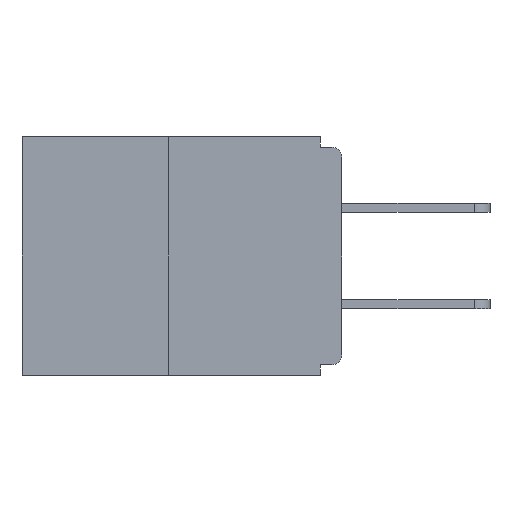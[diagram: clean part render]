
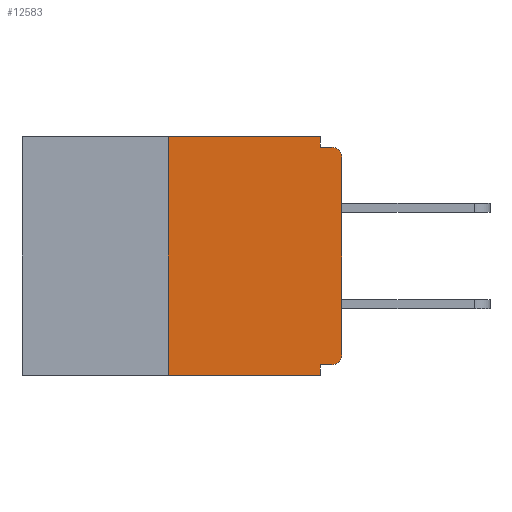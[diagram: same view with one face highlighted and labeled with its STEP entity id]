
A CAD part, left-side view. The second image highlights one B-rep face of the part: STEP entity #12583.
In plain terms, the highlighted planar face has unit normal (-1, 0, 0).
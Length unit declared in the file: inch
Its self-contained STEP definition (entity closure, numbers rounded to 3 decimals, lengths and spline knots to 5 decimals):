
#111 = EDGE_CURVE ( 'NONE', #4546, #5713, #12499, .T. ) ;
#151 = LINE ( 'NONE', #11094, #15594 ) ;
#236 = DIRECTION ( 'NONE',  ( 0., 0., -1. ) ) ;
#401 = EDGE_CURVE ( 'NONE', #11277, #7497, #1067, .T. ) ;
#651 = CARTESIAN_POINT ( 'NONE',  ( 0., 0.25, 0. ) ) ;
#699 = CARTESIAN_POINT ( 'NONE',  ( 0., 0.015, -0.03 ) ) ;
#709 = DIRECTION ( 'NONE',  ( 1., 0., 0. ) ) ;
#753 = DIRECTION ( 'NONE',  ( 0., 0., -1. ) ) ;
#1067 = LINE ( 'NONE', #15602, #11350 ) ;
#1256 = EDGE_CURVE ( 'NONE', #3381, #15644, #15502, .T. ) ;
#1815 = PLANE ( 'NONE',  #13118 ) ;
#2047 = LINE ( 'NONE', #651, #3397 ) ;
#2059 = LINE ( 'NONE', #7414, #3590 ) ;
#2129 = VECTOR ( 'NONE', #236, 39.37008 ) ;
#2247 = DIRECTION ( 'NONE',  ( 0., 1., 0. ) ) ;
#2325 = ORIENTED_EDGE ( 'NONE', *, *, #8929, .T. ) ;
#2362 = LINE ( 'NONE', #3087, #5798 ) ;
#2437 = EDGE_CURVE ( 'NONE', #5713, #10273, #9010, .T. ) ;
#2530 = CARTESIAN_POINT ( 'NONE',  ( 0., 0., -0.03 ) ) ;
#2546 = AXIS2_PLACEMENT_3D ( 'NONE', #699, #5560, #753 ) ;
#2915 = EDGE_CURVE ( 'NONE', #7497, #15644, #15269, .T. ) ;
#3087 = CARTESIAN_POINT ( 'NONE',  ( 0., 0.46, -0.343 ) ) ;
#3180 = ORIENTED_EDGE ( 'NONE', *, *, #3383, .T. ) ;
#3381 = VERTEX_POINT ( 'NONE', #2530 ) ;
#3383 = EDGE_CURVE ( 'NONE', #4546, #11314, #13309, .T. ) ;
#3397 = VECTOR ( 'NONE', #12982, 39.37008 ) ;
#3590 = VECTOR ( 'NONE', #9830, 39.37008 ) ;
#4534 = ORIENTED_EDGE ( 'NONE', *, *, #1256, .T. ) ;
#4546 = VERTEX_POINT ( 'NONE', #8348 ) ;
#4603 = CARTESIAN_POINT ( 'NONE',  ( 0., 0., -0.328 ) ) ;
#4817 = CARTESIAN_POINT ( 'NONE',  ( 0., 0.25, 0. ) ) ;
#5245 = CARTESIAN_POINT ( 'NONE',  ( 0., 0.015, -0.313 ) ) ;
#5555 = VECTOR ( 'NONE', #7659, 39.37008 ) ;
#5560 = DIRECTION ( 'NONE',  ( -1., 0., 0. ) ) ;
#5713 = VERTEX_POINT ( 'NONE', #15294 ) ;
#5798 = VECTOR ( 'NONE', #6676, 39.37008 ) ;
#6578 = EDGE_CURVE ( 'NONE', #13822, #14582, #2047, .T. ) ;
#6600 = ORIENTED_EDGE ( 'NONE', *, *, #111, .F. ) ;
#6676 = DIRECTION ( 'NONE',  ( 0., -1., 0. ) ) ;
#6880 = EDGE_CURVE ( 'NONE', #11314, #3381, #151, .T. ) ;
#7203 = CARTESIAN_POINT ( 'NONE',  ( 0., 0.031, -0.015 ) ) ;
#7414 = CARTESIAN_POINT ( 'NONE',  ( 0., 0.46, 0. ) ) ;
#7482 = CARTESIAN_POINT ( 'NONE',  ( 0., 0., -0.313 ) ) ;
#7497 = VERTEX_POINT ( 'NONE', #7203 ) ;
#7659 = DIRECTION ( 'NONE',  ( 0., -1., 0. ) ) ;
#8340 = VECTOR ( 'NONE', #2247, 39.37008 ) ;
#8348 = CARTESIAN_POINT ( 'NONE',  ( 0., 0.015, -0.328 ) ) ;
#8727 = DIRECTION ( 'NONE',  ( 0., 0., 1. ) ) ;
#8929 = EDGE_CURVE ( 'NONE', #13822, #10273, #2362, .T. ) ;
#9010 = LINE ( 'NONE', #10134, #2129 ) ;
#9643 = EDGE_LOOP ( 'NONE', ( #10672, #15804, #2325, #10410, #6600, #3180, #13299, #4534, #14293, #11371 ) ) ;
#9683 = CARTESIAN_POINT ( 'NONE',  ( 0., 0.031, 0. ) ) ;
#9830 = DIRECTION ( 'NONE',  ( 0., -1., 0. ) ) ;
#10026 = DIRECTION ( 'NONE',  ( -1., 0., 0. ) ) ;
#10134 = CARTESIAN_POINT ( 'NONE',  ( 0., 0.031, -0.343 ) ) ;
#10273 = VERTEX_POINT ( 'NONE', #14820 ) ;
#10388 = DIRECTION ( 'NONE',  ( 0., 0., -1. ) ) ;
#10410 = ORIENTED_EDGE ( 'NONE', *, *, #2437, .F. ) ;
#10672 = ORIENTED_EDGE ( 'NONE', *, *, #13578, .F. ) ;
#11094 = CARTESIAN_POINT ( 'NONE',  ( 0., 0., 0. ) ) ;
#11277 = VERTEX_POINT ( 'NONE', #9683 ) ;
#11314 = VERTEX_POINT ( 'NONE', #7482 ) ;
#11350 = VECTOR ( 'NONE', #13178, 39.37008 ) ;
#11371 = ORIENTED_EDGE ( 'NONE', *, *, #401, .F. ) ;
#11383 = CARTESIAN_POINT ( 'NONE',  ( 0., 0.25, -0.343 ) ) ;
#11485 = CARTESIAN_POINT ( 'NONE',  ( 0., 0.46, 0. ) ) ;
#12499 = LINE ( 'NONE', #4603, #8340 ) ;
#12583 = ADVANCED_FACE ( 'NONE', ( #13435 ), #1815, .F. ) ;
#12982 = DIRECTION ( 'NONE',  ( 0., 0., 1. ) ) ;
#13021 = CARTESIAN_POINT ( 'NONE',  ( 0., 0.015, -0.015 ) ) ;
#13118 = AXIS2_PLACEMENT_3D ( 'NONE', #11485, #709, #10388 ) ;
#13178 = DIRECTION ( 'NONE',  ( 0., 0., -1. ) ) ;
#13299 = ORIENTED_EDGE ( 'NONE', *, *, #6880, .T. ) ;
#13309 = CIRCLE ( 'NONE', #14799, 0.015 ) ;
#13435 = FACE_OUTER_BOUND ( 'NONE', #9643, .T. ) ;
#13578 = EDGE_CURVE ( 'NONE', #14582, #11277, #2059, .T. ) ;
#13635 = DIRECTION ( 'NONE',  ( 0., 0., -1. ) ) ;
#13822 = VERTEX_POINT ( 'NONE', #11383 ) ;
#14293 = ORIENTED_EDGE ( 'NONE', *, *, #2915, .F. ) ;
#14582 = VERTEX_POINT ( 'NONE', #4817 ) ;
#14799 = AXIS2_PLACEMENT_3D ( 'NONE', #5245, #10026, #13635 ) ;
#14820 = CARTESIAN_POINT ( 'NONE',  ( 0., 0.031, -0.343 ) ) ;
#14900 = CARTESIAN_POINT ( 'NONE',  ( 0., 0., -0.015 ) ) ;
#15269 = LINE ( 'NONE', #14900, #5555 ) ;
#15294 = CARTESIAN_POINT ( 'NONE',  ( 0., 0.031, -0.328 ) ) ;
#15502 = CIRCLE ( 'NONE', #2546, 0.015 ) ;
#15594 = VECTOR ( 'NONE', #8727, 39.37008 ) ;
#15602 = CARTESIAN_POINT ( 'NONE',  ( 0., 0.031, 0. ) ) ;
#15644 = VERTEX_POINT ( 'NONE', #13021 ) ;
#15804 = ORIENTED_EDGE ( 'NONE', *, *, #6578, .F. ) ;
